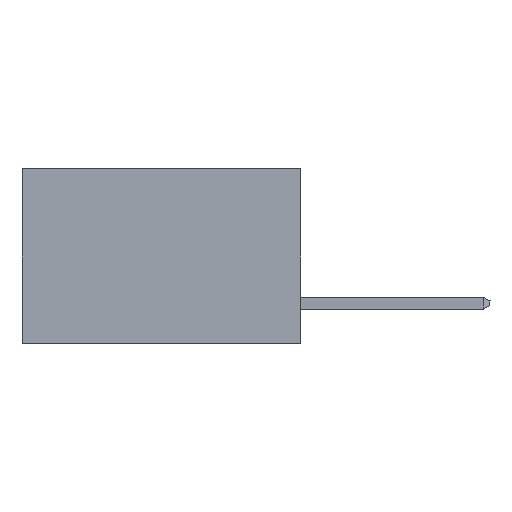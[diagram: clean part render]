
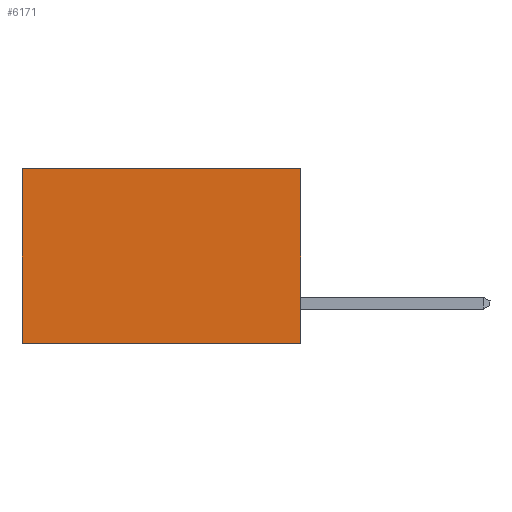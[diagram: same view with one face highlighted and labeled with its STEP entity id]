
A CAD part, left-side view. The second image highlights one B-rep face of the part: STEP entity #6171.
In plain terms, the highlighted planar face has unit normal (-1, 0, 0).
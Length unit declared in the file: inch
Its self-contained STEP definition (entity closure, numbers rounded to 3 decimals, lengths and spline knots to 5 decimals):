
#27 = VERTEX_POINT ( 'NONE', #9114 ) ;
#99 = DIRECTION ( 'NONE',  ( 0., 0., -1. ) ) ;
#561 = EDGE_CURVE ( 'NONE', #27, #4717, #9289, .T. ) ;
#1383 = VERTEX_POINT ( 'NONE', #9581 ) ;
#2916 = CARTESIAN_POINT ( 'NONE',  ( 0.277, 0.59, -0.37 ) ) ;
#3113 = VERTEX_POINT ( 'NONE', #11915 ) ;
#4033 = DIRECTION ( 'NONE',  ( 0., 0., -1. ) ) ;
#4260 = LINE ( 'NONE', #7716, #9698 ) ;
#4682 = ORIENTED_EDGE ( 'NONE', *, *, #10945, .T. ) ;
#4717 = VERTEX_POINT ( 'NONE', #11108 ) ;
#5669 = VECTOR ( 'NONE', #99, 39.37008 ) ;
#5723 = CARTESIAN_POINT ( 'NONE',  ( 0.277, 0., -0.37 ) ) ;
#6171 = ADVANCED_FACE ( 'NONE', ( #11651 ), #13700, .F. ) ;
#6826 = EDGE_LOOP ( 'NONE', ( #4682, #10014, #8047, #9146 ) ) ;
#7309 = DIRECTION ( 'NONE',  ( 0., 1., 0. ) ) ;
#7716 = CARTESIAN_POINT ( 'NONE',  ( 0.277, 0., 0. ) ) ;
#8047 = ORIENTED_EDGE ( 'NONE', *, *, #12545, .F. ) ;
#9114 = CARTESIAN_POINT ( 'NONE',  ( 0.277, 0., -0.37 ) ) ;
#9146 = ORIENTED_EDGE ( 'NONE', *, *, #11808, .T. ) ;
#9289 = LINE ( 'NONE', #5723, #11780 ) ;
#9581 = CARTESIAN_POINT ( 'NONE',  ( 0.277, 0.59, 0. ) ) ;
#9698 = VECTOR ( 'NONE', #10949, 39.37008 ) ;
#10014 = ORIENTED_EDGE ( 'NONE', *, *, #561, .F. ) ;
#10395 = VECTOR ( 'NONE', #4033, 39.37008 ) ;
#10945 = EDGE_CURVE ( 'NONE', #1383, #4717, #13425, .T. ) ;
#10949 = DIRECTION ( 'NONE',  ( 0., 1., 0. ) ) ;
#11108 = CARTESIAN_POINT ( 'NONE',  ( 0.277, 0.59, -0.37 ) ) ;
#11131 = CARTESIAN_POINT ( 'NONE',  ( 0.277, 0., -0.37 ) ) ;
#11385 = LINE ( 'NONE', #11131, #5669 ) ;
#11651 = FACE_OUTER_BOUND ( 'NONE', #6826, .T. ) ;
#11780 = VECTOR ( 'NONE', #7309, 39.37008 ) ;
#11808 = EDGE_CURVE ( 'NONE', #3113, #1383, #4260, .T. ) ;
#11915 = CARTESIAN_POINT ( 'NONE',  ( 0.277, 0., 0. ) ) ;
#12376 = AXIS2_PLACEMENT_3D ( 'NONE', #13653, #13638, #13486 ) ;
#12545 = EDGE_CURVE ( 'NONE', #3113, #27, #11385, .T. ) ;
#13425 = LINE ( 'NONE', #2916, #10395 ) ;
#13486 = DIRECTION ( 'NONE',  ( 0., 0., -1. ) ) ;
#13638 = DIRECTION ( 'NONE',  ( 1., 0., 0. ) ) ;
#13653 = CARTESIAN_POINT ( 'NONE',  ( 0.277, 0., -0.37 ) ) ;
#13700 = PLANE ( 'NONE',  #12376 ) ;
